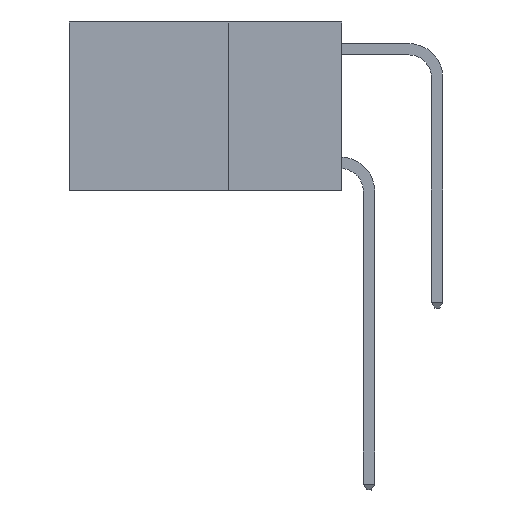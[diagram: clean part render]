
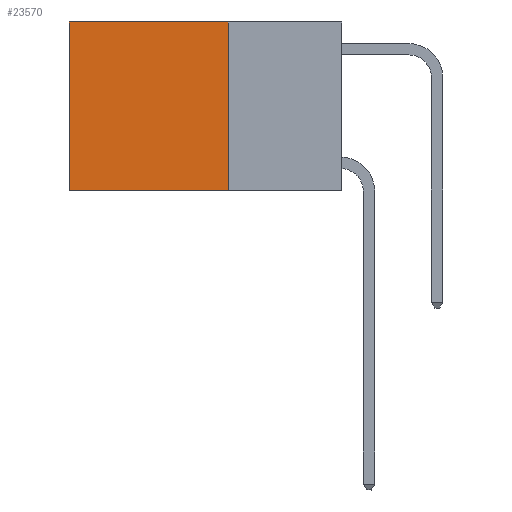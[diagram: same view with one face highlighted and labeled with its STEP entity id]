
A CAD part, left-side view. The second image highlights one B-rep face of the part: STEP entity #23570.
In plain terms, the highlighted planar face has unit normal (-1, 0, 0).
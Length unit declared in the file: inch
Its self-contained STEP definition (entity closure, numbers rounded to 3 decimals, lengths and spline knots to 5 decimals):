
#36 = VECTOR ( 'NONE', #348, 39.37008 ) ;
#348 = DIRECTION ( 'NONE',  ( 0., 0., -1. ) ) ;
#763 = CARTESIAN_POINT ( 'NONE',  ( 0.2625, 0.25, 0. ) ) ;
#1367 = DIRECTION ( 'NONE',  ( 0., 0., -1. ) ) ;
#2586 = EDGE_CURVE ( 'NONE', #20602, #23346, #19070, .T. ) ;
#2626 = CARTESIAN_POINT ( 'NONE',  ( 0.2625, 0.25, -0.37 ) ) ;
#2937 = EDGE_CURVE ( 'NONE', #9338, #14635, #15145, .T. ) ;
#4180 = CARTESIAN_POINT ( 'NONE',  ( 0.2625, 0.25, 0. ) ) ;
#5151 = CARTESIAN_POINT ( 'NONE',  ( 0.2625, 0.6, 0. ) ) ;
#6092 = AXIS2_PLACEMENT_3D ( 'NONE', #763, #10389, #23040 ) ;
#7195 = VECTOR ( 'NONE', #22916, 39.37008 ) ;
#7425 = CARTESIAN_POINT ( 'NONE',  ( 0.2625, 0.6, 0. ) ) ;
#8443 = FACE_OUTER_BOUND ( 'NONE', #20672, .T. ) ;
#9338 = VERTEX_POINT ( 'NONE', #15887 ) ;
#9930 = CARTESIAN_POINT ( 'NONE',  ( 0.2625, 0.6, -0.37 ) ) ;
#10389 = DIRECTION ( 'NONE',  ( 1., 0., 0. ) ) ;
#10507 = LINE ( 'NONE', #5151, #16232 ) ;
#11502 = DIRECTION ( 'NONE',  ( 0., 1., 0. ) ) ;
#13254 = LINE ( 'NONE', #14969, #36 ) ;
#13387 = EDGE_CURVE ( 'NONE', #9338, #20602, #13254, .T. ) ;
#14415 = ORIENTED_EDGE ( 'NONE', *, *, #13387, .F. ) ;
#14635 = VERTEX_POINT ( 'NONE', #7425 ) ;
#14969 = CARTESIAN_POINT ( 'NONE',  ( 0.2625, 0.25, 0. ) ) ;
#15145 = LINE ( 'NONE', #4180, #7195 ) ;
#15633 = PLANE ( 'NONE',  #6092 ) ;
#15887 = CARTESIAN_POINT ( 'NONE',  ( 0.2625, 0.25, 0. ) ) ;
#16232 = VECTOR ( 'NONE', #1367, 39.37008 ) ;
#17797 = CARTESIAN_POINT ( 'NONE',  ( 0.2625, 0.25, -0.37 ) ) ;
#19070 = LINE ( 'NONE', #2626, #20842 ) ;
#20602 = VERTEX_POINT ( 'NONE', #17797 ) ;
#20672 = EDGE_LOOP ( 'NONE', ( #21751, #20718, #14415, #23738 ) ) ;
#20718 = ORIENTED_EDGE ( 'NONE', *, *, #2586, .F. ) ;
#20842 = VECTOR ( 'NONE', #11502, 39.37008 ) ;
#21751 = ORIENTED_EDGE ( 'NONE', *, *, #23752, .T. ) ;
#22916 = DIRECTION ( 'NONE',  ( 0., 1., 0. ) ) ;
#23040 = DIRECTION ( 'NONE',  ( 0., 0., -1. ) ) ;
#23346 = VERTEX_POINT ( 'NONE', #9930 ) ;
#23570 = ADVANCED_FACE ( 'NONE', ( #8443 ), #15633, .F. ) ;
#23738 = ORIENTED_EDGE ( 'NONE', *, *, #2937, .T. ) ;
#23752 = EDGE_CURVE ( 'NONE', #14635, #23346, #10507, .T. ) ;
